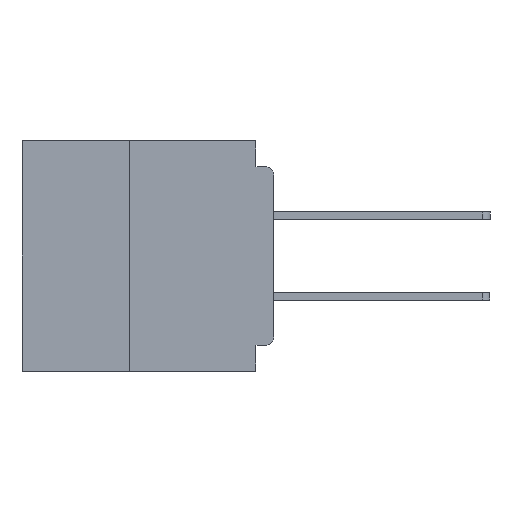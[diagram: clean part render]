
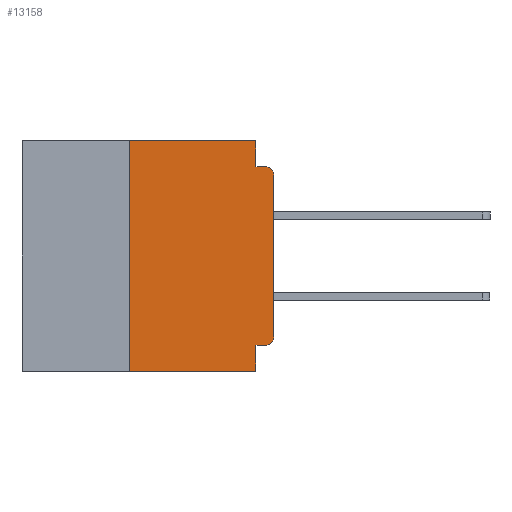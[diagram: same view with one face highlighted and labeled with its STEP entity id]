
A CAD part, left-side view. The second image highlights one B-rep face of the part: STEP entity #13158.
In plain terms, the highlighted planar face has unit normal (-1, 0, 0).
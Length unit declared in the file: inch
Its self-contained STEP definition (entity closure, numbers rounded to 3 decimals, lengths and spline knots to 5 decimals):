
#348 = DIRECTION ( 'NONE',  ( 0., 0., -1. ) ) ;
#913 = DIRECTION ( 'NONE',  ( 0., 0., -1. ) ) ;
#1587 = ORIENTED_EDGE ( 'NONE', *, *, #48946, .F. ) ;
#1681 = VERTEX_POINT ( 'NONE', #43381 ) ;
#2253 = VERTEX_POINT ( 'NONE', #8430 ) ;
#2287 = DIRECTION ( 'NONE',  ( 0., -1., 0. ) ) ;
#4447 = ORIENTED_EDGE ( 'NONE', *, *, #41809, .T. ) ;
#4901 = VECTOR ( 'NONE', #24042, 39.37008 ) ;
#6236 = LINE ( 'NONE', #27376, #24327 ) ;
#6719 = VERTEX_POINT ( 'NONE', #15835 ) ;
#8430 = CARTESIAN_POINT ( 'NONE',  ( 0., 0.031, -0.4 ) ) ;
#9355 = VERTEX_POINT ( 'NONE', #28663 ) ;
#10358 = VERTEX_POINT ( 'NONE', #46208 ) ;
#10375 = CARTESIAN_POINT ( 'NONE',  ( 0., 0., -0.34 ) ) ;
#10698 = ORIENTED_EDGE ( 'NONE', *, *, #35181, .F. ) ;
#10907 = EDGE_CURVE ( 'NONE', #9355, #36894, #6236, .T. ) ;
#11322 = LINE ( 'NONE', #26696, #49645 ) ;
#13158 = ADVANCED_FACE ( 'NONE', ( #25154 ), #15723, .F. ) ;
#13246 = CARTESIAN_POINT ( 'NONE',  ( 0., 0.015, -0.045 ) ) ;
#14821 = DIRECTION ( 'NONE',  ( 0., 1., 0. ) ) ;
#14883 = LINE ( 'NONE', #43567, #44233 ) ;
#15723 = PLANE ( 'NONE',  #16915 ) ;
#15785 = VECTOR ( 'NONE', #39427, 39.37008 ) ;
#15835 = CARTESIAN_POINT ( 'NONE',  ( 0., 0.031, -0.355 ) ) ;
#16354 = LINE ( 'NONE', #43081, #4901 ) ;
#16566 = AXIS2_PLACEMENT_3D ( 'NONE', #46894, #24031, #913 ) ;
#16894 = DIRECTION ( 'NONE',  ( -1., 0., 0. ) ) ;
#16915 = AXIS2_PLACEMENT_3D ( 'NONE', #19604, #23467, #348 ) ;
#17717 = CARTESIAN_POINT ( 'NONE',  ( 0., 0., -0.06 ) ) ;
#18067 = VERTEX_POINT ( 'NONE', #13246 ) ;
#18237 = VERTEX_POINT ( 'NONE', #10375 ) ;
#18443 = ORIENTED_EDGE ( 'NONE', *, *, #43109, .F. ) ;
#18533 = CARTESIAN_POINT ( 'NONE',  ( 0., 0., -0.355 ) ) ;
#18564 = LINE ( 'NONE', #44732, #35393 ) ;
#19488 = ORIENTED_EDGE ( 'NONE', *, *, #29707, .F. ) ;
#19604 = CARTESIAN_POINT ( 'NONE',  ( 0., 0.437, 0. ) ) ;
#20965 = ORIENTED_EDGE ( 'NONE', *, *, #37514, .T. ) ;
#21540 = CARTESIAN_POINT ( 'NONE',  ( 0., 0.437, -0.4 ) ) ;
#21865 = DIRECTION ( 'NONE',  ( 0., 0., 1. ) ) ;
#23467 = DIRECTION ( 'NONE',  ( 1., 0., 0. ) ) ;
#24031 = DIRECTION ( 'NONE',  ( -1., 0., 0. ) ) ;
#24042 = DIRECTION ( 'NONE',  ( 0., 0., 1. ) ) ;
#24327 = VECTOR ( 'NONE', #31205, 39.37008 ) ;
#24699 = VERTEX_POINT ( 'NONE', #17717 ) ;
#25154 = FACE_OUTER_BOUND ( 'NONE', #43098, .T. ) ;
#26490 = ORIENTED_EDGE ( 'NONE', *, *, #30961, .T. ) ;
#26696 = CARTESIAN_POINT ( 'NONE',  ( 0., 0.031, -0.4 ) ) ;
#27376 = CARTESIAN_POINT ( 'NONE',  ( 0., 0.437, 0. ) ) ;
#28640 = VECTOR ( 'NONE', #2287, 39.37008 ) ;
#28663 = CARTESIAN_POINT ( 'NONE',  ( 0., 0.25, 0. ) ) ;
#29707 = EDGE_CURVE ( 'NONE', #6719, #2253, #11322, .T. ) ;
#30624 = CIRCLE ( 'NONE', #16566, 0.015 ) ;
#30793 = LINE ( 'NONE', #18533, #39731 ) ;
#30961 = EDGE_CURVE ( 'NONE', #1681, #18237, #30624, .T. ) ;
#31205 = DIRECTION ( 'NONE',  ( 0., -1., 0. ) ) ;
#35181 = EDGE_CURVE ( 'NONE', #1681, #6719, #30793, .T. ) ;
#35249 = AXIS2_PLACEMENT_3D ( 'NONE', #39879, #16894, #43678 ) ;
#35393 = VECTOR ( 'NONE', #21865, 39.37008 ) ;
#35591 = CARTESIAN_POINT ( 'NONE',  ( 0., 0., -0.045 ) ) ;
#35951 = VERTEX_POINT ( 'NONE', #38603 ) ;
#36894 = VERTEX_POINT ( 'NONE', #41009 ) ;
#37514 = EDGE_CURVE ( 'NONE', #18237, #24699, #18564, .T. ) ;
#38042 = ORIENTED_EDGE ( 'NONE', *, *, #10907, .F. ) ;
#38603 = CARTESIAN_POINT ( 'NONE',  ( 0., 0.25, -0.4 ) ) ;
#39174 = CIRCLE ( 'NONE', #35249, 0.015 ) ;
#39427 = DIRECTION ( 'NONE',  ( 0., -1., 0. ) ) ;
#39731 = VECTOR ( 'NONE', #14821, 39.37008 ) ;
#39879 = CARTESIAN_POINT ( 'NONE',  ( 0., 0.015, -0.06 ) ) ;
#39987 = LINE ( 'NONE', #21540, #28640 ) ;
#41009 = CARTESIAN_POINT ( 'NONE',  ( 0., 0.031, 0. ) ) ;
#41809 = EDGE_CURVE ( 'NONE', #24699, #18067, #39174, .T. ) ;
#42122 = ORIENTED_EDGE ( 'NONE', *, *, #44341, .T. ) ;
#43081 = CARTESIAN_POINT ( 'NONE',  ( 0., 0.25, -0.4 ) ) ;
#43098 = EDGE_LOOP ( 'NONE', ( #20965, #4447, #1587, #18443, #38042, #48693, #42122, #19488, #10698, #26490 ) ) ;
#43109 = EDGE_CURVE ( 'NONE', #36894, #10358, #14883, .T. ) ;
#43381 = CARTESIAN_POINT ( 'NONE',  ( 0., 0.015, -0.355 ) ) ;
#43567 = CARTESIAN_POINT ( 'NONE',  ( 0., 0.031, 0. ) ) ;
#43678 = DIRECTION ( 'NONE',  ( 0., 0., -1. ) ) ;
#44233 = VECTOR ( 'NONE', #47398, 39.37008 ) ;
#44341 = EDGE_CURVE ( 'NONE', #35951, #2253, #39987, .T. ) ;
#44732 = CARTESIAN_POINT ( 'NONE',  ( 0., 0., 0. ) ) ;
#45841 = DIRECTION ( 'NONE',  ( 0., 0., -1. ) ) ;
#46208 = CARTESIAN_POINT ( 'NONE',  ( 0., 0.031, -0.045 ) ) ;
#46338 = LINE ( 'NONE', #35591, #15785 ) ;
#46894 = CARTESIAN_POINT ( 'NONE',  ( 0., 0.015, -0.34 ) ) ;
#47030 = EDGE_CURVE ( 'NONE', #35951, #9355, #16354, .T. ) ;
#47398 = DIRECTION ( 'NONE',  ( 0., 0., -1. ) ) ;
#48693 = ORIENTED_EDGE ( 'NONE', *, *, #47030, .F. ) ;
#48946 = EDGE_CURVE ( 'NONE', #10358, #18067, #46338, .T. ) ;
#49645 = VECTOR ( 'NONE', #45841, 39.37008 ) ;
